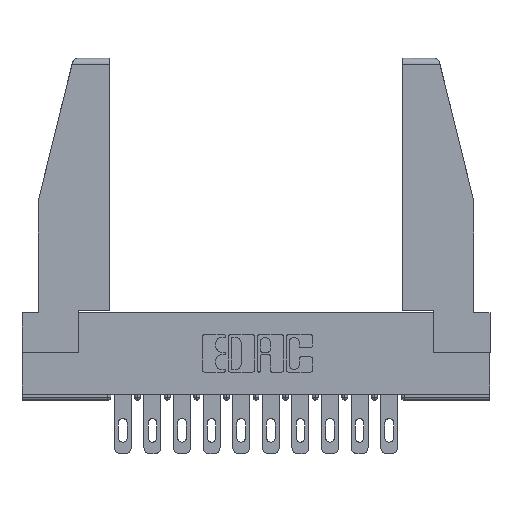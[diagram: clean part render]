
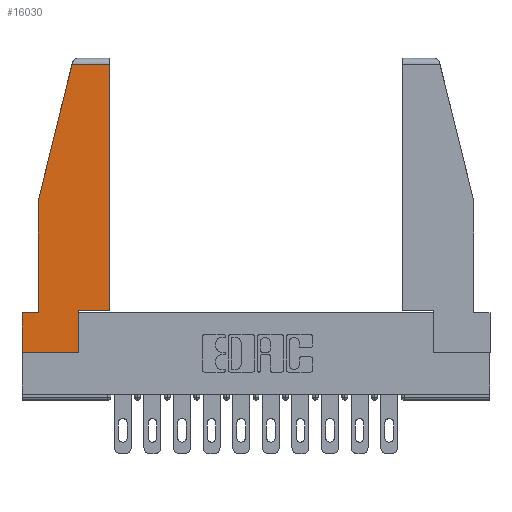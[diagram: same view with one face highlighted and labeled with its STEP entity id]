
A CAD part, top view. The second image highlights one B-rep face of the part: STEP entity #16030.
In plain terms, the highlighted planar face has unit normal (0, 0, 1).
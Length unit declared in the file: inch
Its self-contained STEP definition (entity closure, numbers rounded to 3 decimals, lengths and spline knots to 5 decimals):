
#390 = DIRECTION ( 'NONE',  ( 0., 0., 1. ) ) ;
#525 = VECTOR ( 'NONE', #1223, 39.37008 ) ;
#1100 = CARTESIAN_POINT ( 'NONE',  ( 0., 1.52, 0. ) ) ;
#1223 = DIRECTION ( 'NONE',  ( 1., 0., 0. ) ) ;
#1290 = LINE ( 'NONE', #17089, #10247 ) ;
#1531 = DIRECTION ( 'NONE',  ( 0., 1., 0. ) ) ;
#1711 = VECTOR ( 'NONE', #15752, 39.37008 ) ;
#1999 = LINE ( 'NONE', #3222, #8864 ) ;
#2038 = ORIENTED_EDGE ( 'NONE', *, *, #6859, .T. ) ;
#2417 = FACE_OUTER_BOUND ( 'NONE', #12710, .T. ) ;
#3076 = CARTESIAN_POINT ( 'NONE',  ( 0.2636, 1.52, 0. ) ) ;
#3222 = CARTESIAN_POINT ( 'NONE',  ( 0.086, 0.8, 0. ) ) ;
#3279 = DIRECTION ( 'NONE',  ( 0., -1., 0. ) ) ;
#3305 = EDGE_CURVE ( 'NONE', #15391, #5232, #9207, .T. ) ;
#3358 = EDGE_CURVE ( 'NONE', #10668, #4484, #1290, .T. ) ;
#3496 = EDGE_CURVE ( 'NONE', #5232, #16089, #14785, .T. ) ;
#3616 = ORIENTED_EDGE ( 'NONE', *, *, #11447, .T. ) ;
#3745 = CARTESIAN_POINT ( 'NONE',  ( 0., 0.21, 0. ) ) ;
#3748 = ORIENTED_EDGE ( 'NONE', *, *, #5239, .T. ) ;
#4025 = CARTESIAN_POINT ( 'NONE',  ( 0., 0.21, 0. ) ) ;
#4203 = CARTESIAN_POINT ( 'NONE',  ( 0., 0., 0. ) ) ;
#4208 = VECTOR ( 'NONE', #5504, 39.37008 ) ;
#4484 = VERTEX_POINT ( 'NONE', #9711 ) ;
#4536 = AXIS2_PLACEMENT_3D ( 'NONE', #12300, #390, #13752 ) ;
#4947 = ORIENTED_EDGE ( 'NONE', *, *, #3358, .T. ) ;
#5088 = ORIENTED_EDGE ( 'NONE', *, *, #3496, .T. ) ;
#5232 = VERTEX_POINT ( 'NONE', #10087 ) ;
#5239 = EDGE_CURVE ( 'NONE', #15576, #15391, #12528, .T. ) ;
#5504 = DIRECTION ( 'NONE',  ( 1., 0., 0. ) ) ;
#5595 = ORIENTED_EDGE ( 'NONE', *, *, #10376, .T. ) ;
#5733 = CARTESIAN_POINT ( 'NONE',  ( 0.086, 0.21, 0. ) ) ;
#6001 = DIRECTION ( 'NONE',  ( -1., 0., 0. ) ) ;
#6323 = VECTOR ( 'NONE', #6001, 39.37008 ) ;
#6584 = LINE ( 'NONE', #14520, #525 ) ;
#6700 = ORIENTED_EDGE ( 'NONE', *, *, #9016, .T. ) ;
#6859 = EDGE_CURVE ( 'NONE', #17121, #15608, #14975, .T. ) ;
#7178 = CARTESIAN_POINT ( 'NONE',  ( 0.461, 1.52, 0. ) ) ;
#7651 = ORIENTED_EDGE ( 'NONE', *, *, #3305, .T. ) ;
#8065 = CARTESIAN_POINT ( 'NONE',  ( 0.461, 0.223, 0. ) ) ;
#8635 = CARTESIAN_POINT ( 'NONE',  ( 0.297, 0.223, 0. ) ) ;
#8864 = VECTOR ( 'NONE', #3279, 39.37008 ) ;
#9016 = EDGE_CURVE ( 'NONE', #4484, #15576, #1999, .T. ) ;
#9055 = LINE ( 'NONE', #1100, #9881 ) ;
#9207 = LINE ( 'NONE', #3745, #1711 ) ;
#9240 = EDGE_CURVE ( 'NONE', #11389, #17121, #6584, .T. ) ;
#9696 = PLANE ( 'NONE',  #4536 ) ;
#9711 = CARTESIAN_POINT ( 'NONE',  ( 0.086, 0.8, 0. ) ) ;
#9881 = VECTOR ( 'NONE', #14352, 39.37008 ) ;
#10087 = CARTESIAN_POINT ( 'NONE',  ( 0., 0., 0. ) ) ;
#10247 = VECTOR ( 'NONE', #11867, 39.37008 ) ;
#10376 = EDGE_CURVE ( 'NONE', #15608, #10668, #9055, .T. ) ;
#10668 = VERTEX_POINT ( 'NONE', #3076 ) ;
#11389 = VERTEX_POINT ( 'NONE', #8635 ) ;
#11447 = EDGE_CURVE ( 'NONE', #16089, #11389, #14789, .T. ) ;
#11867 = DIRECTION ( 'NONE',  ( -0.239, -0.971, 0. ) ) ;
#12300 = CARTESIAN_POINT ( 'NONE',  ( 0., 0., 0. ) ) ;
#12528 = LINE ( 'NONE', #12530, #6323 ) ;
#12530 = CARTESIAN_POINT ( 'NONE',  ( 0., 0.21, 0. ) ) ;
#12710 = EDGE_LOOP ( 'NONE', ( #2038, #5595, #4947, #6700, #3748, #7651, #5088, #3616, #14816 ) ) ;
#12808 = CARTESIAN_POINT ( 'NONE',  ( 0.297, 0., 0. ) ) ;
#13634 = CARTESIAN_POINT ( 'NONE',  ( 0.297, 0., 0. ) ) ;
#13752 = DIRECTION ( 'NONE',  ( 1., 0., 0. ) ) ;
#14141 = VECTOR ( 'NONE', #1531, 39.37008 ) ;
#14187 = VECTOR ( 'NONE', #16763, 39.37008 ) ;
#14352 = DIRECTION ( 'NONE',  ( -1., 0., 0. ) ) ;
#14520 = CARTESIAN_POINT ( 'NONE',  ( 0.297, 0.223, 0. ) ) ;
#14785 = LINE ( 'NONE', #4203, #4208 ) ;
#14789 = LINE ( 'NONE', #12808, #14187 ) ;
#14816 = ORIENTED_EDGE ( 'NONE', *, *, #9240, .T. ) ;
#14975 = LINE ( 'NONE', #8065, #14141 ) ;
#15054 = CARTESIAN_POINT ( 'NONE',  ( 0.461, 0.223, 0. ) ) ;
#15391 = VERTEX_POINT ( 'NONE', #4025 ) ;
#15576 = VERTEX_POINT ( 'NONE', #5733 ) ;
#15608 = VERTEX_POINT ( 'NONE', #7178 ) ;
#15752 = DIRECTION ( 'NONE',  ( 0., -1., 0. ) ) ;
#16030 = ADVANCED_FACE ( 'NONE', ( #2417 ), #9696, .T. ) ;
#16089 = VERTEX_POINT ( 'NONE', #13634 ) ;
#16763 = DIRECTION ( 'NONE',  ( 0., 1., 0. ) ) ;
#17089 = CARTESIAN_POINT ( 'NONE',  ( 0.271, 1.55, 0. ) ) ;
#17121 = VERTEX_POINT ( 'NONE', #15054 ) ;
